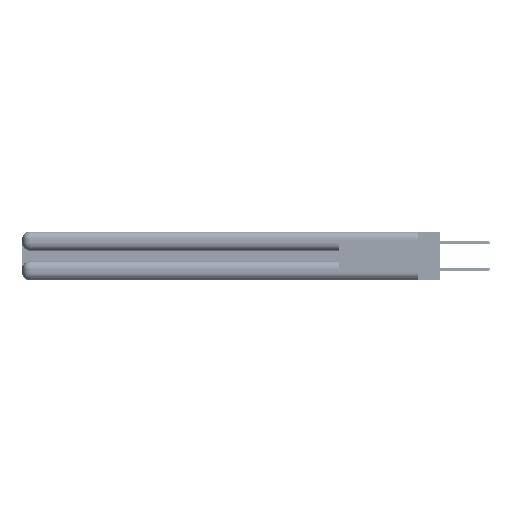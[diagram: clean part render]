
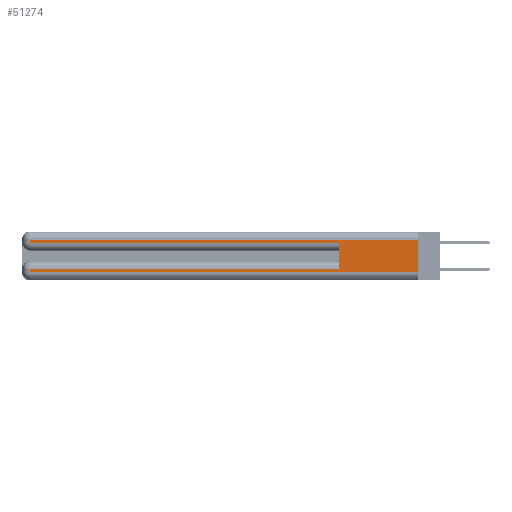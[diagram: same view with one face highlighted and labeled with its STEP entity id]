
A CAD part, left-side view. The second image highlights one B-rep face of the part: STEP entity #51274.
In plain terms, the highlighted planar face has unit normal (-1, 0, 0).
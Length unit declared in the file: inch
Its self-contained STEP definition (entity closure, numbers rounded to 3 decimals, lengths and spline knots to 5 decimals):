
#666 = ORIENTED_EDGE ( 'NONE', *, *, #2637, .T. ) ;
#2637 = EDGE_CURVE ( 'NONE', #7160, #14842, #38242, .T. ) ;
#3392 = CARTESIAN_POINT ( 'NONE',  ( 0., 0., 0.37 ) ) ;
#3763 = DIRECTION ( 'NONE',  ( 0., 0., 1. ) ) ;
#3981 = EDGE_CURVE ( 'NONE', #43261, #40072, #9157, .T. ) ;
#4083 = VECTOR ( 'NONE', #15632, 39.37008 ) ;
#4328 = DIRECTION ( 'NONE',  ( 0., 0., -1. ) ) ;
#5242 = LINE ( 'NONE', #17027, #50230 ) ;
#5359 = FACE_OUTER_BOUND ( 'NONE', #23061, .T. ) ;
#5674 = DIRECTION ( 'NONE',  ( 0., 0., -1. ) ) ;
#6515 = VECTOR ( 'NONE', #40561, 39.37008 ) ;
#7160 = VERTEX_POINT ( 'NONE', #11977 ) ;
#7406 = VECTOR ( 'NONE', #4328, 39.37008 ) ;
#7582 = DIRECTION ( 'NONE',  ( 0., 0., -1. ) ) ;
#8035 = ORIENTED_EDGE ( 'NONE', *, *, #25622, .F. ) ;
#8084 = ORIENTED_EDGE ( 'NONE', *, *, #3981, .F. ) ;
#9157 = LINE ( 'NONE', #44755, #17509 ) ;
#9819 = VECTOR ( 'NONE', #5674, 39.37008 ) ;
#10478 = VERTEX_POINT ( 'NONE', #32579 ) ;
#11977 = CARTESIAN_POINT ( 'NONE',  ( 0., 2.94, 0.085 ) ) ;
#13658 = CARTESIAN_POINT ( 'NONE',  ( 0., 0., 0.06 ) ) ;
#13675 = LINE ( 'NONE', #41421, #23322 ) ;
#14842 = VERTEX_POINT ( 'NONE', #44076 ) ;
#15632 = DIRECTION ( 'NONE',  ( 0., 0., -1. ) ) ;
#17027 = CARTESIAN_POINT ( 'NONE',  ( 0., 0., 0.285 ) ) ;
#17116 = AXIS2_PLACEMENT_3D ( 'NONE', #3392, #32218, #7582 ) ;
#17509 = VECTOR ( 'NONE', #3763, 39.37008 ) ;
#20733 = LINE ( 'NONE', #26214, #9819 ) ;
#20866 = CARTESIAN_POINT ( 'NONE',  ( 0., 2.94, 0.285 ) ) ;
#20931 = LINE ( 'NONE', #37297, #7406 ) ;
#20937 = DIRECTION ( 'NONE',  ( 0., 1., 0. ) ) ;
#20989 = LINE ( 'NONE', #40248, #30669 ) ;
#21987 = EDGE_CURVE ( 'NONE', #14842, #29682, #20989, .T. ) ;
#23061 = EDGE_LOOP ( 'NONE', ( #8035, #37668, #42171, #52445, #8084, #35634, #666, #42011 ) ) ;
#23322 = VECTOR ( 'NONE', #20937, 39.37008 ) ;
#25362 = CARTESIAN_POINT ( 'NONE',  ( 0., 0., 0.31 ) ) ;
#25622 = EDGE_CURVE ( 'NONE', #42697, #29682, #20931, .T. ) ;
#26214 = CARTESIAN_POINT ( 'NONE',  ( 0., 2.94, 0.37 ) ) ;
#27446 = EDGE_CURVE ( 'NONE', #10478, #46404, #20733, .T. ) ;
#27775 = EDGE_CURVE ( 'NONE', #42697, #10478, #28454, .T. ) ;
#28012 = CARTESIAN_POINT ( 'NONE',  ( 0., 0., 0.31 ) ) ;
#28127 = PLANE ( 'NONE',  #17116 ) ;
#28454 = LINE ( 'NONE', #28012, #6515 ) ;
#28746 = CARTESIAN_POINT ( 'NONE',  ( 0., 0.6, 0.085 ) ) ;
#29682 = VERTEX_POINT ( 'NONE', #13658 ) ;
#30669 = VECTOR ( 'NONE', #52353, 39.37008 ) ;
#32218 = DIRECTION ( 'NONE',  ( 1., 0., 0. ) ) ;
#32579 = CARTESIAN_POINT ( 'NONE',  ( 0., 2.94, 0.31 ) ) ;
#35634 = ORIENTED_EDGE ( 'NONE', *, *, #37118, .T. ) ;
#37118 = EDGE_CURVE ( 'NONE', #43261, #7160, #13675, .T. ) ;
#37297 = CARTESIAN_POINT ( 'NONE',  ( 0., 0., 0.37 ) ) ;
#37668 = ORIENTED_EDGE ( 'NONE', *, *, #27775, .T. ) ;
#38242 = LINE ( 'NONE', #44524, #4083 ) ;
#40072 = VERTEX_POINT ( 'NONE', #44181 ) ;
#40248 = CARTESIAN_POINT ( 'NONE',  ( 0., 0., 0.06 ) ) ;
#40561 = DIRECTION ( 'NONE',  ( 0., 1., 0. ) ) ;
#41421 = CARTESIAN_POINT ( 'NONE',  ( 0., 0., 0.085 ) ) ;
#42011 = ORIENTED_EDGE ( 'NONE', *, *, #21987, .T. ) ;
#42171 = ORIENTED_EDGE ( 'NONE', *, *, #27446, .T. ) ;
#42697 = VERTEX_POINT ( 'NONE', #25362 ) ;
#43261 = VERTEX_POINT ( 'NONE', #28746 ) ;
#44076 = CARTESIAN_POINT ( 'NONE',  ( 0., 2.94, 0.06 ) ) ;
#44181 = CARTESIAN_POINT ( 'NONE',  ( 0., 0.6, 0.285 ) ) ;
#44524 = CARTESIAN_POINT ( 'NONE',  ( 0., 2.94, 0.37 ) ) ;
#44755 = CARTESIAN_POINT ( 'NONE',  ( 0., 0.6, 0.145 ) ) ;
#45717 = DIRECTION ( 'NONE',  ( 0., -1., 0. ) ) ;
#46404 = VERTEX_POINT ( 'NONE', #20866 ) ;
#48409 = EDGE_CURVE ( 'NONE', #46404, #40072, #5242, .T. ) ;
#50230 = VECTOR ( 'NONE', #45717, 39.37008 ) ;
#51274 = ADVANCED_FACE ( 'NONE', ( #5359 ), #28127, .F. ) ;
#52353 = DIRECTION ( 'NONE',  ( 0., -1., 0. ) ) ;
#52445 = ORIENTED_EDGE ( 'NONE', *, *, #48409, .T. ) ;
